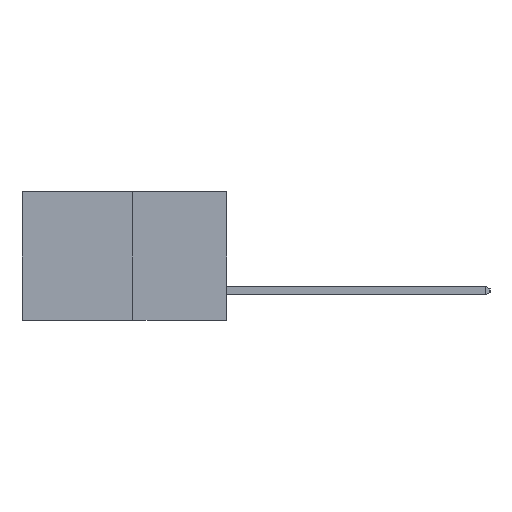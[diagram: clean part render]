
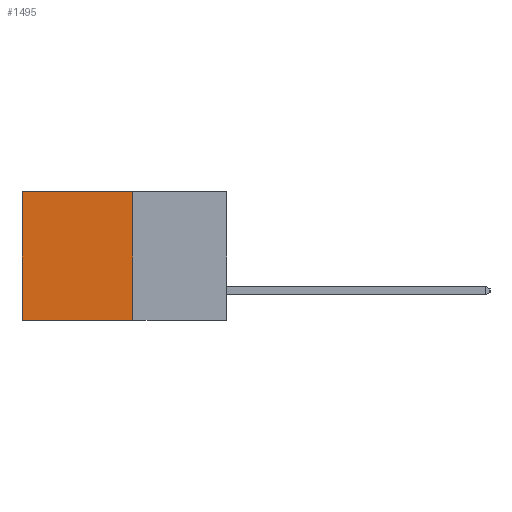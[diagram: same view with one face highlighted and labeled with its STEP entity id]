
A CAD part, left-side view. The second image highlights one B-rep face of the part: STEP entity #1495.
In plain terms, the highlighted planar face has unit normal (-1, 0, 0).
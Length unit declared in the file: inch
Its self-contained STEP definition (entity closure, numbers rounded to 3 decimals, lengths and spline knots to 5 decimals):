
#163 = PLANE ( 'NONE',  #5115 ) ;
#358 = VERTEX_POINT ( 'NONE', #10315 ) ;
#584 = LINE ( 'NONE', #1782, #13671 ) ;
#646 = DIRECTION ( 'NONE',  ( 0., 1., 0. ) ) ;
#805 = CARTESIAN_POINT ( 'NONE',  ( 0.277, 0.27, -0.37 ) ) ;
#948 = VERTEX_POINT ( 'NONE', #10975 ) ;
#970 = DIRECTION ( 'NONE',  ( 1., 0., 0. ) ) ;
#1495 = ADVANCED_FACE ( 'NONE', ( #6854 ), #163, .F. ) ;
#1782 = CARTESIAN_POINT ( 'NONE',  ( 0.277, 0.27, 0. ) ) ;
#1984 = ORIENTED_EDGE ( 'NONE', *, *, #12131, .T. ) ;
#2371 = EDGE_LOOP ( 'NONE', ( #1984, #10610, #9552, #5567 ) ) ;
#2492 = VECTOR ( 'NONE', #646, 39.37008 ) ;
#2742 = DIRECTION ( 'NONE',  ( 0., 0., -1. ) ) ;
#2821 = VERTEX_POINT ( 'NONE', #8783 ) ;
#2882 = VECTOR ( 'NONE', #3561, 39.37008 ) ;
#2963 = VECTOR ( 'NONE', #13091, 39.37008 ) ;
#3561 = DIRECTION ( 'NONE',  ( 0., 0., -1. ) ) ;
#4627 = CARTESIAN_POINT ( 'NONE',  ( 0.277, 0.27, -0.37 ) ) ;
#5115 = AXIS2_PLACEMENT_3D ( 'NONE', #805, #970, #2742 ) ;
#5567 = ORIENTED_EDGE ( 'NONE', *, *, #12333, .T. ) ;
#5795 = LINE ( 'NONE', #4627, #2882 ) ;
#6854 = FACE_OUTER_BOUND ( 'NONE', #2371, .T. ) ;
#6876 = CARTESIAN_POINT ( 'NONE',  ( 0.277, 0.59, -0.37 ) ) ;
#8140 = VERTEX_POINT ( 'NONE', #13572 ) ;
#8224 = LINE ( 'NONE', #13358, #2492 ) ;
#8783 = CARTESIAN_POINT ( 'NONE',  ( 0.277, 0.59, 0. ) ) ;
#9552 = ORIENTED_EDGE ( 'NONE', *, *, #10906, .F. ) ;
#10315 = CARTESIAN_POINT ( 'NONE',  ( 0.277, 0.27, -0.37 ) ) ;
#10610 = ORIENTED_EDGE ( 'NONE', *, *, #11668, .F. ) ;
#10906 = EDGE_CURVE ( 'NONE', #948, #358, #5795, .T. ) ;
#10975 = CARTESIAN_POINT ( 'NONE',  ( 0.277, 0.27, 0. ) ) ;
#11107 = LINE ( 'NONE', #6876, #2963 ) ;
#11668 = EDGE_CURVE ( 'NONE', #358, #8140, #8224, .T. ) ;
#12131 = EDGE_CURVE ( 'NONE', #2821, #8140, #11107, .T. ) ;
#12333 = EDGE_CURVE ( 'NONE', #948, #2821, #584, .T. ) ;
#12416 = DIRECTION ( 'NONE',  ( 0., 1., 0. ) ) ;
#13091 = DIRECTION ( 'NONE',  ( 0., 0., -1. ) ) ;
#13358 = CARTESIAN_POINT ( 'NONE',  ( 0.277, 0.27, -0.37 ) ) ;
#13572 = CARTESIAN_POINT ( 'NONE',  ( 0.277, 0.59, -0.37 ) ) ;
#13671 = VECTOR ( 'NONE', #12416, 39.37008 ) ;
